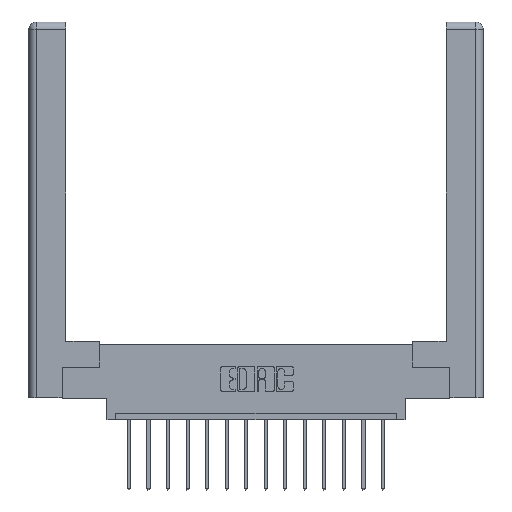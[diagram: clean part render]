
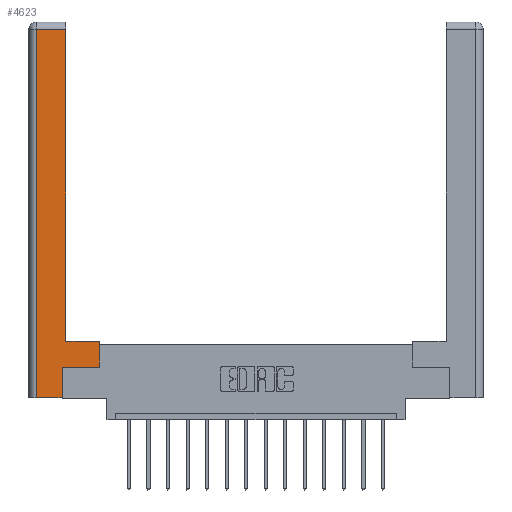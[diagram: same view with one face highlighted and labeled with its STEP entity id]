
A CAD part, top view. The second image highlights one B-rep face of the part: STEP entity #4623.
In plain terms, the highlighted planar face has unit normal (0, 0, 1).
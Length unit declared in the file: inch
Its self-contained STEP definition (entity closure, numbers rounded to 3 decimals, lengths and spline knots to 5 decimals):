
#178 = CARTESIAN_POINT ( 'NONE',  ( 0.295, 0.45, 0. ) ) ;
#243 = EDGE_CURVE ( 'NONE', #1346, #7946, #14696, .T. ) ;
#289 = EDGE_CURVE ( 'NONE', #15792, #1346, #11009, .T. ) ;
#856 = CARTESIAN_POINT ( 'NONE',  ( 0.265, 0.245, 0. ) ) ;
#902 = EDGE_LOOP ( 'NONE', ( #5317, #15955, #8797, #10634, #5740, #14354, #2348, #7499 ) ) ;
#993 = VERTEX_POINT ( 'NONE', #5845 ) ;
#1201 = CARTESIAN_POINT ( 'NONE',  ( 0.565, 0.45, 0. ) ) ;
#1346 = VERTEX_POINT ( 'NONE', #9115 ) ;
#1957 = VECTOR ( 'NONE', #4563, 39.37008 ) ;
#2348 = ORIENTED_EDGE ( 'NONE', *, *, #243, .T. ) ;
#2590 = VERTEX_POINT ( 'NONE', #7187 ) ;
#2603 = DIRECTION ( 'NONE',  ( 0., 1., 0. ) ) ;
#2761 = DIRECTION ( 'NONE',  ( -1., 0., 0. ) ) ;
#2894 = LINE ( 'NONE', #856, #12031 ) ;
#3094 = VECTOR ( 'NONE', #2603, 39.37008 ) ;
#3141 = DIRECTION ( 'NONE',  ( 0., 1., 0. ) ) ;
#3349 = CARTESIAN_POINT ( 'NONE',  ( 0.565, 0.45, 0. ) ) ;
#3356 = DIRECTION ( 'NONE',  ( 0., 0., -1. ) ) ;
#3636 = EDGE_CURVE ( 'NONE', #7946, #15270, #10504, .T. ) ;
#3859 = DIRECTION ( 'NONE',  ( -1., 0., 0. ) ) ;
#4249 = VECTOR ( 'NONE', #15477, 39.37008 ) ;
#4563 = DIRECTION ( 'NONE',  ( 1., 0., 0. ) ) ;
#4623 = ADVANCED_FACE ( 'NONE', ( #5641 ), #9928, .F. ) ;
#4877 = VECTOR ( 'NONE', #3141, 39.37008 ) ;
#5317 = ORIENTED_EDGE ( 'NONE', *, *, #13552, .T. ) ;
#5641 = FACE_OUTER_BOUND ( 'NONE', #902, .T. ) ;
#5740 = ORIENTED_EDGE ( 'NONE', *, *, #11807, .T. ) ;
#5845 = CARTESIAN_POINT ( 'NONE',  ( 0.265, 0., 0. ) ) ;
#6069 = DIRECTION ( 'NONE',  ( 0., 1., 0. ) ) ;
#7148 = CARTESIAN_POINT ( 'NONE',  ( 0.295, 2.94, 0. ) ) ;
#7187 = CARTESIAN_POINT ( 'NONE',  ( 0.0615, 0., 0. ) ) ;
#7397 = VECTOR ( 'NONE', #3859, 39.37008 ) ;
#7499 = ORIENTED_EDGE ( 'NONE', *, *, #3636, .T. ) ;
#7946 = VERTEX_POINT ( 'NONE', #3349 ) ;
#8316 = CARTESIAN_POINT ( 'NONE',  ( 0.295, 3., 0. ) ) ;
#8697 = CARTESIAN_POINT ( 'NONE',  ( 0.295, 0.45, 0. ) ) ;
#8797 = ORIENTED_EDGE ( 'NONE', *, *, #14906, .T. ) ;
#8808 = VECTOR ( 'NONE', #2761, 39.37008 ) ;
#9115 = CARTESIAN_POINT ( 'NONE',  ( 0.565, 0.245, 0. ) ) ;
#9218 = CARTESIAN_POINT ( 'NONE',  ( 0.0615, 2.94, 0. ) ) ;
#9533 = DIRECTION ( 'NONE',  ( 1., 0., 0. ) ) ;
#9928 = PLANE ( 'NONE',  #11423 ) ;
#10063 = LINE ( 'NONE', #11014, #1957 ) ;
#10504 = LINE ( 'NONE', #178, #8808 ) ;
#10510 = CARTESIAN_POINT ( 'NONE',  ( 0.0615, 0., 0. ) ) ;
#10634 = ORIENTED_EDGE ( 'NONE', *, *, #16736, .T. ) ;
#10826 = LINE ( 'NONE', #9218, #7397 ) ;
#11009 = LINE ( 'NONE', #13404, #13881 ) ;
#11014 = CARTESIAN_POINT ( 'NONE',  ( 0.265, 0., 0. ) ) ;
#11190 = VERTEX_POINT ( 'NONE', #7148 ) ;
#11348 = EDGE_CURVE ( 'NONE', #11190, #11418, #10826, .T. ) ;
#11418 = VERTEX_POINT ( 'NONE', #13144 ) ;
#11423 = AXIS2_PLACEMENT_3D ( 'NONE', #12390, #3356, #12443 ) ;
#11758 = LINE ( 'NONE', #8316, #4877 ) ;
#11807 = EDGE_CURVE ( 'NONE', #993, #15792, #2894, .T. ) ;
#12031 = VECTOR ( 'NONE', #6069, 39.37008 ) ;
#12390 = CARTESIAN_POINT ( 'NONE',  ( 0., 0., 0. ) ) ;
#12443 = DIRECTION ( 'NONE',  ( -1., 0., 0. ) ) ;
#12456 = CARTESIAN_POINT ( 'NONE',  ( 0.265, 0.245, 0. ) ) ;
#13144 = CARTESIAN_POINT ( 'NONE',  ( 0.0615, 2.94, 0. ) ) ;
#13404 = CARTESIAN_POINT ( 'NONE',  ( 0.565, 0.245, 0. ) ) ;
#13552 = EDGE_CURVE ( 'NONE', #15270, #11190, #11758, .T. ) ;
#13881 = VECTOR ( 'NONE', #9533, 39.37008 ) ;
#14354 = ORIENTED_EDGE ( 'NONE', *, *, #289, .T. ) ;
#14631 = LINE ( 'NONE', #10510, #4249 ) ;
#14696 = LINE ( 'NONE', #1201, #3094 ) ;
#14906 = EDGE_CURVE ( 'NONE', #11418, #2590, #14631, .T. ) ;
#15270 = VERTEX_POINT ( 'NONE', #8697 ) ;
#15477 = DIRECTION ( 'NONE',  ( 0., -1., 0. ) ) ;
#15792 = VERTEX_POINT ( 'NONE', #12456 ) ;
#15955 = ORIENTED_EDGE ( 'NONE', *, *, #11348, .T. ) ;
#16736 = EDGE_CURVE ( 'NONE', #2590, #993, #10063, .T. ) ;
